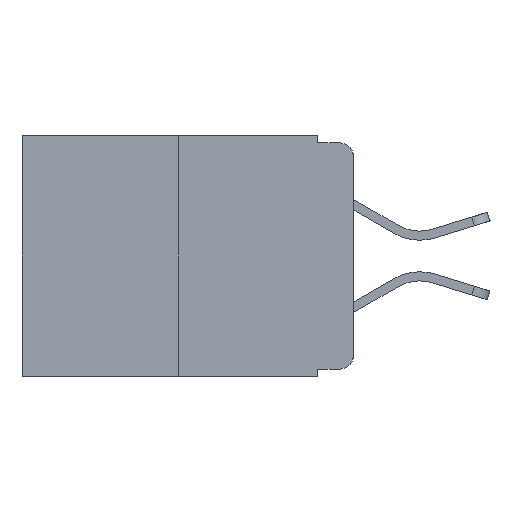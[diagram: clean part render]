
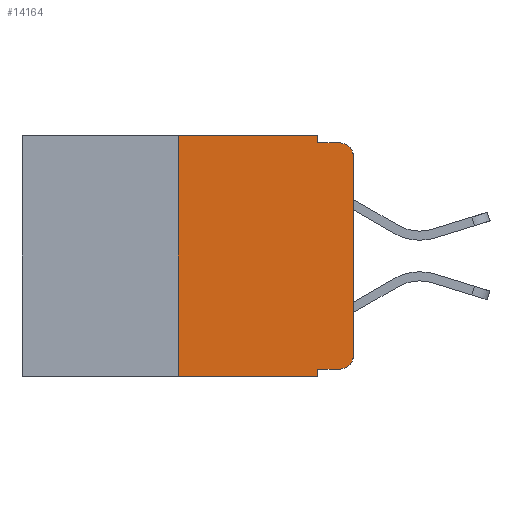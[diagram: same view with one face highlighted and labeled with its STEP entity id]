
A CAD part, left-side view. The second image highlights one B-rep face of the part: STEP entity #14164.
In plain terms, the highlighted planar face has unit normal (-1, 0, 0).
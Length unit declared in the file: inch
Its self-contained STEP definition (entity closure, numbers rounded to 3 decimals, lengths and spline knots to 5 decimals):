
#1 = EDGE_CURVE ( 'NONE', #12971, #8428, #6305, .T. ) ;
#3 = EDGE_CURVE ( 'NONE', #7254, #3504, #12742, .T. ) ;
#145 = CARTESIAN_POINT ( 'NONE',  ( 0., 0.473, -0.343 ) ) ;
#638 = CARTESIAN_POINT ( 'NONE',  ( 0., 0.02, -0.333 ) ) ;
#664 = DIRECTION ( 'NONE',  ( 0., 0., -1. ) ) ;
#1109 = EDGE_CURVE ( 'NONE', #7254, #7633, #7054, .T. ) ;
#1126 = DIRECTION ( 'NONE',  ( 0., 0., 1. ) ) ;
#1336 = EDGE_LOOP ( 'NONE', ( #14504, #11766, #2194, #9009, #3098, #6906, #10478, #4297, #10844, #13972 ) ) ;
#1961 = LINE ( 'NONE', #5208, #11582 ) ;
#2153 = EDGE_CURVE ( 'NONE', #6812, #12971, #3820, .T. ) ;
#2194 = ORIENTED_EDGE ( 'NONE', *, *, #3987, .F. ) ;
#2436 = CARTESIAN_POINT ( 'NONE',  ( 0., 0.051, 0. ) ) ;
#2897 = VECTOR ( 'NONE', #10867, 39.37008 ) ;
#3098 = ORIENTED_EDGE ( 'NONE', *, *, #1, .F. ) ;
#3127 = EDGE_CURVE ( 'NONE', #8428, #10502, #6387, .T. ) ;
#3249 = DIRECTION ( 'NONE',  ( 0., -1., 0. ) ) ;
#3485 = CARTESIAN_POINT ( 'NONE',  ( 0., 0.473, 0. ) ) ;
#3504 = VERTEX_POINT ( 'NONE', #638 ) ;
#3820 = LINE ( 'NONE', #5406, #16248 ) ;
#3987 = EDGE_CURVE ( 'NONE', #10502, #13895, #11846, .T. ) ;
#4234 = CIRCLE ( 'NONE', #12278, 0.02 ) ;
#4297 = ORIENTED_EDGE ( 'NONE', *, *, #1109, .F. ) ;
#4754 = CARTESIAN_POINT ( 'NONE',  ( 0., 0.25, -0.343 ) ) ;
#4815 = EDGE_CURVE ( 'NONE', #13930, #13895, #12211, .T. ) ;
#4962 = DIRECTION ( 'NONE',  ( 0., 0., 1. ) ) ;
#5208 = CARTESIAN_POINT ( 'NONE',  ( 0., 0., 0. ) ) ;
#5272 = CARTESIAN_POINT ( 'NONE',  ( 0., 0.02, -0.01 ) ) ;
#5406 = CARTESIAN_POINT ( 'NONE',  ( 0., 0.25, 0. ) ) ;
#5601 = CARTESIAN_POINT ( 'NONE',  ( 0., 0.02, -0.03 ) ) ;
#5764 = DIRECTION ( 'NONE',  ( 1., 0., 0. ) ) ;
#5862 = DIRECTION ( 'NONE',  ( 0., -1., 0. ) ) ;
#6305 = LINE ( 'NONE', #3485, #2897 ) ;
#6387 = LINE ( 'NONE', #6773, #15189 ) ;
#6498 = CARTESIAN_POINT ( 'NONE',  ( 0., 0.051, -0.333 ) ) ;
#6543 = EDGE_CURVE ( 'NONE', #12236, #13930, #1961, .T. ) ;
#6615 = CARTESIAN_POINT ( 'NONE',  ( 0., 0., -0.03 ) ) ;
#6651 = VECTOR ( 'NONE', #8485, 39.37008 ) ;
#6773 = CARTESIAN_POINT ( 'NONE',  ( 0., 0.051, 0. ) ) ;
#6812 = VERTEX_POINT ( 'NONE', #4754 ) ;
#6897 = DIRECTION ( 'NONE',  ( 0., 0., -1. ) ) ;
#6906 = ORIENTED_EDGE ( 'NONE', *, *, #2153, .F. ) ;
#7054 = LINE ( 'NONE', #15309, #6651 ) ;
#7207 = CARTESIAN_POINT ( 'NONE',  ( 0., 0.051, -0.343 ) ) ;
#7254 = VERTEX_POINT ( 'NONE', #6498 ) ;
#7336 = CARTESIAN_POINT ( 'NONE',  ( 0., 0.051, -0.01 ) ) ;
#7359 = CARTESIAN_POINT ( 'NONE',  ( 0., 0., -0.313 ) ) ;
#7633 = VERTEX_POINT ( 'NONE', #7207 ) ;
#8003 = CARTESIAN_POINT ( 'NONE',  ( 0., 0.051, -0.01 ) ) ;
#8209 = DIRECTION ( 'NONE',  ( 0., -1., 0. ) ) ;
#8247 = CARTESIAN_POINT ( 'NONE',  ( 0., 0.473, 0. ) ) ;
#8428 = VERTEX_POINT ( 'NONE', #2436 ) ;
#8465 = DIRECTION ( 'NONE',  ( 0., 0., -1. ) ) ;
#8468 = AXIS2_PLACEMENT_3D ( 'NONE', #8247, #5764, #14166 ) ;
#8485 = DIRECTION ( 'NONE',  ( 0., 0., -1. ) ) ;
#8634 = DIRECTION ( 'NONE',  ( -1., 0., 0. ) ) ;
#8697 = VECTOR ( 'NONE', #8209, 39.37008 ) ;
#9009 = ORIENTED_EDGE ( 'NONE', *, *, #3127, .F. ) ;
#10478 = ORIENTED_EDGE ( 'NONE', *, *, #12710, .T. ) ;
#10502 = VERTEX_POINT ( 'NONE', #7336 ) ;
#10613 = PLANE ( 'NONE',  #8468 ) ;
#10844 = ORIENTED_EDGE ( 'NONE', *, *, #3, .T. ) ;
#10867 = DIRECTION ( 'NONE',  ( 0., -1., 0. ) ) ;
#11582 = VECTOR ( 'NONE', #1126, 39.37008 ) ;
#11766 = ORIENTED_EDGE ( 'NONE', *, *, #4815, .T. ) ;
#11846 = LINE ( 'NONE', #8003, #8697 ) ;
#12211 = CIRCLE ( 'NONE', #15772, 0.02 ) ;
#12223 = CARTESIAN_POINT ( 'NONE',  ( 0., 0.25, 0. ) ) ;
#12236 = VERTEX_POINT ( 'NONE', #7359 ) ;
#12278 = AXIS2_PLACEMENT_3D ( 'NONE', #15701, #8634, #664 ) ;
#12371 = VECTOR ( 'NONE', #5862, 39.37008 ) ;
#12710 = EDGE_CURVE ( 'NONE', #6812, #7633, #13828, .T. ) ;
#12742 = LINE ( 'NONE', #16073, #12371 ) ;
#12971 = VERTEX_POINT ( 'NONE', #12223 ) ;
#13492 = VECTOR ( 'NONE', #3249, 39.37008 ) ;
#13828 = LINE ( 'NONE', #145, #13492 ) ;
#13895 = VERTEX_POINT ( 'NONE', #5272 ) ;
#13930 = VERTEX_POINT ( 'NONE', #6615 ) ;
#13962 = FACE_OUTER_BOUND ( 'NONE', #1336, .T. ) ;
#13972 = ORIENTED_EDGE ( 'NONE', *, *, #15636, .T. ) ;
#14016 = DIRECTION ( 'NONE',  ( -1., 0., 0. ) ) ;
#14164 = ADVANCED_FACE ( 'NONE', ( #13962 ), #10613, .F. ) ;
#14166 = DIRECTION ( 'NONE',  ( 0., 0., -1. ) ) ;
#14504 = ORIENTED_EDGE ( 'NONE', *, *, #6543, .T. ) ;
#15189 = VECTOR ( 'NONE', #8465, 39.37008 ) ;
#15309 = CARTESIAN_POINT ( 'NONE',  ( 0., 0.051, 0. ) ) ;
#15636 = EDGE_CURVE ( 'NONE', #3504, #12236, #4234, .T. ) ;
#15701 = CARTESIAN_POINT ( 'NONE',  ( 0., 0.02, -0.313 ) ) ;
#15772 = AXIS2_PLACEMENT_3D ( 'NONE', #5601, #14016, #6897 ) ;
#16073 = CARTESIAN_POINT ( 'NONE',  ( 0., 0.051, -0.333 ) ) ;
#16248 = VECTOR ( 'NONE', #4962, 39.37008 ) ;
